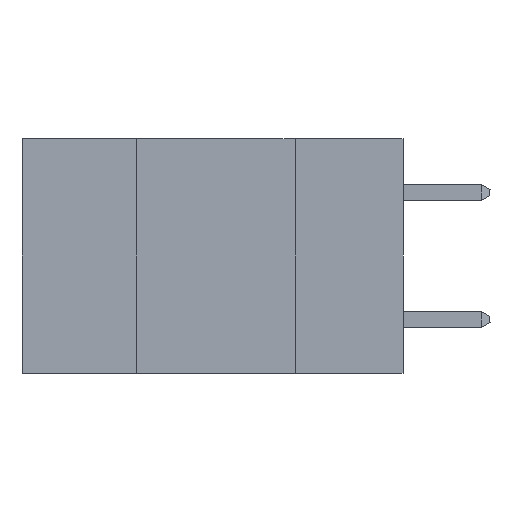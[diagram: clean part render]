
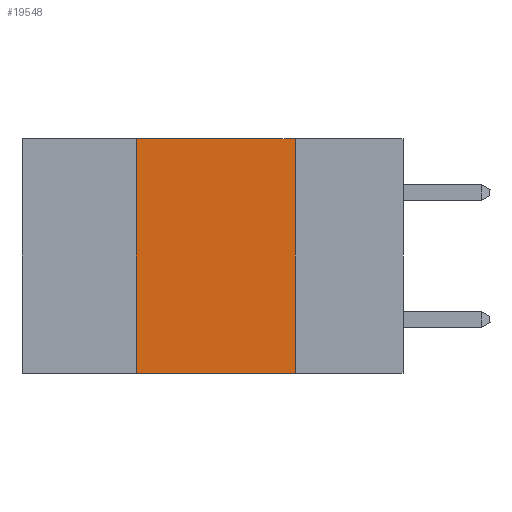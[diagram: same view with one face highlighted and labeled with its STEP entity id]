
A CAD part, left-side view. The second image highlights one B-rep face of the part: STEP entity #19548.
In plain terms, the highlighted planar face has unit normal (-1, 0, 0).
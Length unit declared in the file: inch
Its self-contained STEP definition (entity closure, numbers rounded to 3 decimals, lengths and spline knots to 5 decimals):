
#1678 = FACE_OUTER_BOUND ( 'NONE', #20894, .T. ) ;
#1978 = CARTESIAN_POINT ( 'NONE',  ( 0., 0.6, 0. ) ) ;
#1993 = VECTOR ( 'NONE', #17676, 39.37008 ) ;
#2106 = CARTESIAN_POINT ( 'NONE',  ( 0., 0.6, -0.37 ) ) ;
#3256 = VECTOR ( 'NONE', #5972, 39.37008 ) ;
#3367 = ORIENTED_EDGE ( 'NONE', *, *, #22794, .F. ) ;
#3902 = DIRECTION ( 'NONE',  ( 1., 0., 0. ) ) ;
#4299 = EDGE_CURVE ( 'NONE', #24206, #8878, #6413, .T. ) ;
#5051 = VERTEX_POINT ( 'NONE', #11979 ) ;
#5747 = DIRECTION ( 'NONE',  ( 0., 0., -1. ) ) ;
#5972 = DIRECTION ( 'NONE',  ( 0., -1., 0. ) ) ;
#6413 = LINE ( 'NONE', #2106, #3256 ) ;
#8878 = VERTEX_POINT ( 'NONE', #20968 ) ;
#9447 = EDGE_CURVE ( 'NONE', #24206, #5051, #24585, .T. ) ;
#11423 = ORIENTED_EDGE ( 'NONE', *, *, #20335, .F. ) ;
#11585 = CARTESIAN_POINT ( 'NONE',  ( 0., 0.17, 0. ) ) ;
#11979 = CARTESIAN_POINT ( 'NONE',  ( 0., 0.42, 0. ) ) ;
#12849 = CARTESIAN_POINT ( 'NONE',  ( 0., 0.42, 0. ) ) ;
#13363 = VECTOR ( 'NONE', #18771, 39.37008 ) ;
#15320 = CARTESIAN_POINT ( 'NONE',  ( 0., 0.42, -0.37 ) ) ;
#15381 = ORIENTED_EDGE ( 'NONE', *, *, #4299, .T. ) ;
#17676 = DIRECTION ( 'NONE',  ( 0., -1., 0. ) ) ;
#18523 = AXIS2_PLACEMENT_3D ( 'NONE', #1978, #3902, #5747 ) ;
#18771 = DIRECTION ( 'NONE',  ( 0., 0., 1. ) ) ;
#19146 = VECTOR ( 'NONE', #23760, 39.37008 ) ;
#19417 = CARTESIAN_POINT ( 'NONE',  ( 0., 0.6, 0. ) ) ;
#19548 = ADVANCED_FACE ( 'NONE', ( #1678 ), #23352, .F. ) ;
#19811 = LINE ( 'NONE', #19417, #1993 ) ;
#20335 = EDGE_CURVE ( 'NONE', #24250, #8878, #21313, .T. ) ;
#20894 = EDGE_LOOP ( 'NONE', ( #11423, #3367, #23070, #15381 ) ) ;
#20968 = CARTESIAN_POINT ( 'NONE',  ( 0., 0.17, -0.37 ) ) ;
#21313 = LINE ( 'NONE', #25764, #19146 ) ;
#22794 = EDGE_CURVE ( 'NONE', #5051, #24250, #19811, .T. ) ;
#23070 = ORIENTED_EDGE ( 'NONE', *, *, #9447, .F. ) ;
#23352 = PLANE ( 'NONE',  #18523 ) ;
#23760 = DIRECTION ( 'NONE',  ( 0., 0., -1. ) ) ;
#24206 = VERTEX_POINT ( 'NONE', #15320 ) ;
#24250 = VERTEX_POINT ( 'NONE', #11585 ) ;
#24585 = LINE ( 'NONE', #12849, #13363 ) ;
#25764 = CARTESIAN_POINT ( 'NONE',  ( 0., 0.17, 0. ) ) ;
